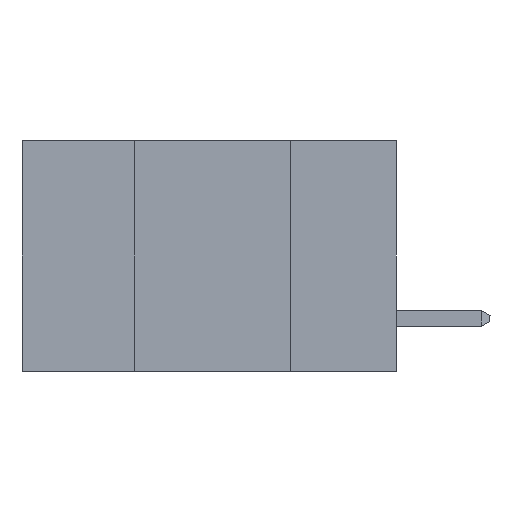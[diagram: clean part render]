
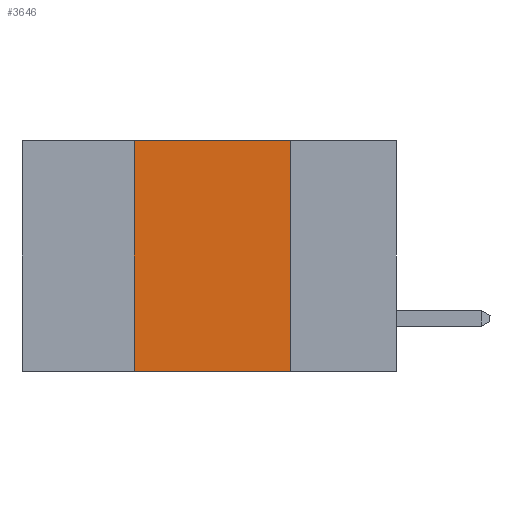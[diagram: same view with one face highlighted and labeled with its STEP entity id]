
A CAD part, left-side view. The second image highlights one B-rep face of the part: STEP entity #3646.
In plain terms, the highlighted planar face has unit normal (-1, 0, 0).
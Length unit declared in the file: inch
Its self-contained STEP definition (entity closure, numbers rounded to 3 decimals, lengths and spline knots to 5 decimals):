
#2408 = LINE ( 'NONE', #18613, #12953 ) ;
#3500 = VERTEX_POINT ( 'NONE', #15868 ) ;
#3646 = ADVANCED_FACE ( 'NONE', ( #6647 ), #17996, .F. ) ;
#4262 = CARTESIAN_POINT ( 'NONE',  ( 0., 0.17, -0.37 ) ) ;
#4385 = VECTOR ( 'NONE', #12018, 39.37008 ) ;
#4956 = DIRECTION ( 'NONE',  ( 0., -1., 0. ) ) ;
#5250 = VECTOR ( 'NONE', #4956, 39.37008 ) ;
#5275 = VECTOR ( 'NONE', #18888, 39.37008 ) ;
#6205 = VERTEX_POINT ( 'NONE', #20671 ) ;
#6647 = FACE_OUTER_BOUND ( 'NONE', #17122, .T. ) ;
#6865 = DIRECTION ( 'NONE',  ( 1., 0., 0. ) ) ;
#6945 = CARTESIAN_POINT ( 'NONE',  ( 0., 0.17, 0. ) ) ;
#7523 = CARTESIAN_POINT ( 'NONE',  ( 0., 0.42, -0.37 ) ) ;
#7696 = CARTESIAN_POINT ( 'NONE',  ( 0., 0.42, 0. ) ) ;
#7980 = ORIENTED_EDGE ( 'NONE', *, *, #8130, .F. ) ;
#8130 = EDGE_CURVE ( 'NONE', #20584, #20697, #14718, .T. ) ;
#8471 = DIRECTION ( 'NONE',  ( 0., 0., -1. ) ) ;
#8993 = ORIENTED_EDGE ( 'NONE', *, *, #20411, .F. ) ;
#9361 = EDGE_CURVE ( 'NONE', #6205, #20584, #11062, .T. ) ;
#10068 = ORIENTED_EDGE ( 'NONE', *, *, #16456, .T. ) ;
#11062 = LINE ( 'NONE', #7523, #5275 ) ;
#12018 = DIRECTION ( 'NONE',  ( 0., 0., -1. ) ) ;
#12953 = VECTOR ( 'NONE', #16995, 39.37008 ) ;
#13618 = ORIENTED_EDGE ( 'NONE', *, *, #9361, .F. ) ;
#14718 = LINE ( 'NONE', #19663, #5250 ) ;
#15868 = CARTESIAN_POINT ( 'NONE',  ( 0., 0.17, -0.37 ) ) ;
#16456 = EDGE_CURVE ( 'NONE', #6205, #3500, #2408, .T. ) ;
#16995 = DIRECTION ( 'NONE',  ( 0., -1., 0. ) ) ;
#17122 = EDGE_LOOP ( 'NONE', ( #8993, #7980, #13618, #10068 ) ) ;
#17996 = PLANE ( 'NONE',  #18710 ) ;
#18428 = CARTESIAN_POINT ( 'NONE',  ( 0., 0.6, 0. ) ) ;
#18613 = CARTESIAN_POINT ( 'NONE',  ( 0., 0.6, -0.37 ) ) ;
#18710 = AXIS2_PLACEMENT_3D ( 'NONE', #18428, #6865, #8471 ) ;
#18888 = DIRECTION ( 'NONE',  ( 0., 0., 1. ) ) ;
#19663 = CARTESIAN_POINT ( 'NONE',  ( 0., 0.6, 0. ) ) ;
#20280 = LINE ( 'NONE', #4262, #4385 ) ;
#20411 = EDGE_CURVE ( 'NONE', #20697, #3500, #20280, .T. ) ;
#20584 = VERTEX_POINT ( 'NONE', #7696 ) ;
#20671 = CARTESIAN_POINT ( 'NONE',  ( 0., 0.42, -0.37 ) ) ;
#20697 = VERTEX_POINT ( 'NONE', #6945 ) ;
